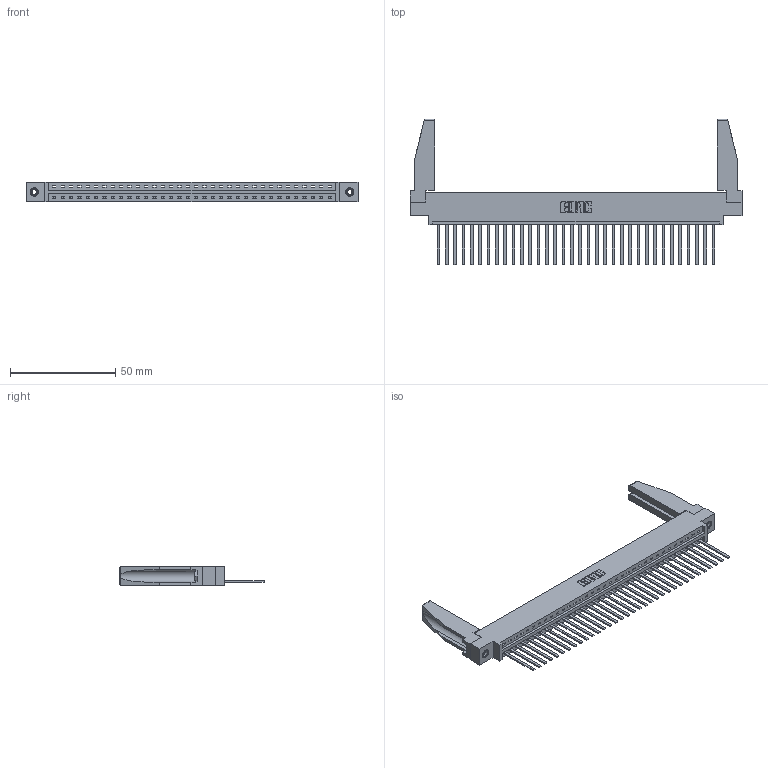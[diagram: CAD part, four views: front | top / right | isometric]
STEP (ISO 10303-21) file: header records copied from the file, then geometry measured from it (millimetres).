
FILE_DESCRIPTION (( 'STEP AP203' ), '1' );
FILE_NAME ('387-034-544-678.STEP', '2019-10-04T11:37:53', ( '' ), ( '' ), 'SwSTEP 2.0', 'SolidWorks 2016', '' );
FILE_SCHEMA (( 'CONFIG_CONTROL_DESIGN' ));
Length unit declared in the file: inch
Products named in the file (5): 337 Part_0.170 Offset - 0.156 Dia-TI; 307-220-078; 345-292-001_345-293-144; 345-250-001_345-250-001-102; 387-034-544-678
Assembly tree (39 placements, depth 2):
  387-034-544-678
    337 Part_0.170 Offset - 0.156 Dia-TI
    345-292-001_345-293-144  x34
    345-250-001_345-250-001-102  x2
    307-220-078  x2
Bounding box: 157.73 x 69.09 x 9.4 mm (x, y, z)
Volume: 20563.3 mm3; surface area: 22306.8 mm2
Topology: 39 solids, 39 shells, 2152 faces, 6433 edges, 4234 vertices
Faces by surface type: plane 1586, cylinder 550, cone 12, torus 4
Entity records: 28696 total; most frequent: CARTESIAN_POINT 4990, ORIENTED_EDGE 4916, DIRECTION 4222, EDGE_CURVE 2458, LINE 2296, VECTOR 2296, VERTEX_POINT 1632, AXIS2_PLACEMENT_3D 963
